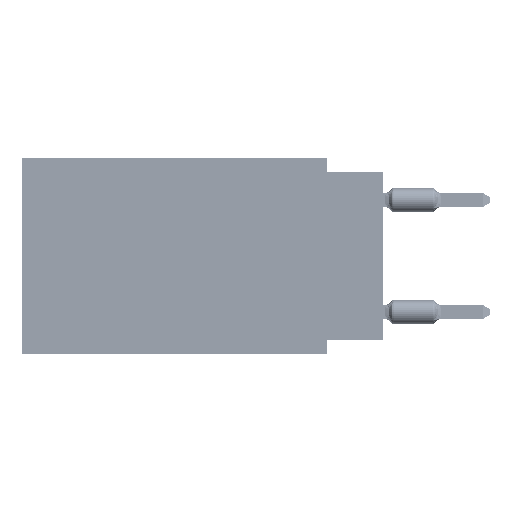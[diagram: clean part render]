
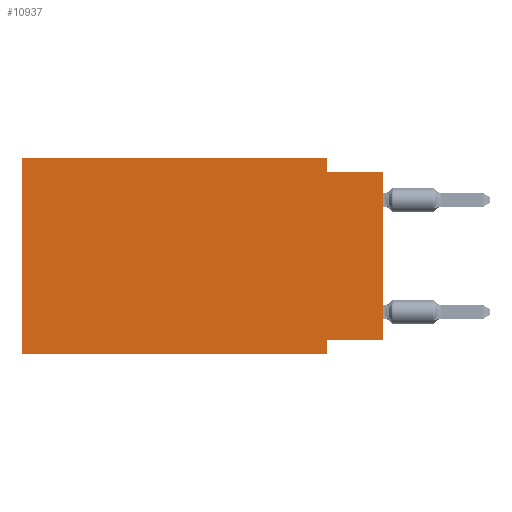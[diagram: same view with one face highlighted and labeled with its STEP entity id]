
A CAD part, left-side view. The second image highlights one B-rep face of the part: STEP entity #10937.
In plain terms, the highlighted planar face has unit normal (-1, 0, 0).
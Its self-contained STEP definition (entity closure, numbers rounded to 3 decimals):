
#2096 = EDGE_CURVE ( 'NONE', #69413, #49470, #41511, .T. ) ;
#5150 = VERTEX_POINT ( 'NONE', #9041 ) ;
#8595 = ORIENTED_EDGE ( 'NONE', *, *, #33761, .F. ) ;
#9041 = CARTESIAN_POINT ( 'NONE',  ( 0., 2.54, 0. ) ) ;
#9292 = CARTESIAN_POINT ( 'NONE',  ( 0., 2.54, -8.89 ) ) ;
#10937 = ADVANCED_FACE ( 'NONE', ( #19559 ), #19094, .F. ) ;
#11481 = DIRECTION ( 'NONE',  ( 0., -1., 0. ) ) ;
#13439 = EDGE_CURVE ( 'NONE', #59198, #5150, #77782, .T. ) ;
#15055 = DIRECTION ( 'NONE',  ( 0., -1., 0. ) ) ;
#19094 = PLANE ( 'NONE',  #81210 ) ;
#19559 = FACE_OUTER_BOUND ( 'NONE', #87181, .T. ) ;
#19826 = ORIENTED_EDGE ( 'NONE', *, *, #53532, .F. ) ;
#23833 = LINE ( 'NONE', #9292, #80689 ) ;
#25296 = EDGE_CURVE ( 'NONE', #86383, #49470, #42517, .T. ) ;
#27376 = CARTESIAN_POINT ( 'NONE',  ( 0., 2.54, -8.255 ) ) ;
#29003 = CARTESIAN_POINT ( 'NONE',  ( 0., 16.383, 0. ) ) ;
#30068 = ORIENTED_EDGE ( 'NONE', *, *, #61194, .F. ) ;
#30643 = CARTESIAN_POINT ( 'NONE',  ( 0., 16.383, 0. ) ) ;
#30698 = ORIENTED_EDGE ( 'NONE', *, *, #2096, .F. ) ;
#33761 = EDGE_CURVE ( 'NONE', #83936, #74518, #23833, .T. ) ;
#34122 = DIRECTION ( 'NONE',  ( 1., 0., 0. ) ) ;
#34676 = VECTOR ( 'NONE', #11481, 1000. ) ;
#35141 = VECTOR ( 'NONE', #36048, 1000. ) ;
#35944 = VECTOR ( 'NONE', #39991, 1000. ) ;
#36048 = DIRECTION ( 'NONE',  ( 0., -1., 0. ) ) ;
#36939 = LINE ( 'NONE', #51019, #76910 ) ;
#37911 = DIRECTION ( 'NONE',  ( 0., 0., -1. ) ) ;
#38393 = ORIENTED_EDGE ( 'NONE', *, *, #88947, .T. ) ;
#39991 = DIRECTION ( 'NONE',  ( 0., 0., 1. ) ) ;
#40229 = DIRECTION ( 'NONE',  ( 0., 0., -1. ) ) ;
#41511 = LINE ( 'NONE', #68247, #34676 ) ;
#42517 = LINE ( 'NONE', #62228, #92619 ) ;
#44725 = ORIENTED_EDGE ( 'NONE', *, *, #52318, .F. ) ;
#48160 = VECTOR ( 'NONE', #15055, 1000. ) ;
#48427 = CARTESIAN_POINT ( 'NONE',  ( 0., 2.54, -0.635 ) ) ;
#49470 = VERTEX_POINT ( 'NONE', #79750 ) ;
#49771 = CARTESIAN_POINT ( 'NONE',  ( 0., 0., -8.255 ) ) ;
#50237 = LINE ( 'NONE', #49771, #53106 ) ;
#51019 = CARTESIAN_POINT ( 'NONE',  ( 0., 2.54, 0. ) ) ;
#52318 = EDGE_CURVE ( 'NONE', #5150, #69413, #36939, .T. ) ;
#53106 = VECTOR ( 'NONE', #78336, 1000. ) ;
#53532 = EDGE_CURVE ( 'NONE', #86383, #83936, #50237, .T. ) ;
#53616 = LINE ( 'NONE', #30643, #35944 ) ;
#57539 = CARTESIAN_POINT ( 'NONE',  ( 0., 16.383, -8.89 ) ) ;
#59198 = VERTEX_POINT ( 'NONE', #62801 ) ;
#61194 = EDGE_CURVE ( 'NONE', #89259, #59198, #53616, .T. ) ;
#62228 = CARTESIAN_POINT ( 'NONE',  ( 0., 0., 0. ) ) ;
#62705 = CARTESIAN_POINT ( 'NONE',  ( 0., 0., -8.255 ) ) ;
#62801 = CARTESIAN_POINT ( 'NONE',  ( 0., 16.383, 0. ) ) ;
#63164 = DIRECTION ( 'NONE',  ( 0., 0., 1. ) ) ;
#65543 = DIRECTION ( 'NONE',  ( 0., 0., -1. ) ) ;
#68247 = CARTESIAN_POINT ( 'NONE',  ( 0., 0., -0.635 ) ) ;
#69280 = CARTESIAN_POINT ( 'NONE',  ( 0., 16.383, 0. ) ) ;
#69413 = VERTEX_POINT ( 'NONE', #48427 ) ;
#74518 = VERTEX_POINT ( 'NONE', #82343 ) ;
#76461 = ORIENTED_EDGE ( 'NONE', *, *, #13439, .F. ) ;
#76910 = VECTOR ( 'NONE', #65543, 1000. ) ;
#77782 = LINE ( 'NONE', #29003, #35141 ) ;
#78336 = DIRECTION ( 'NONE',  ( 0., 1., 0. ) ) ;
#79293 = LINE ( 'NONE', #85858, #48160 ) ;
#79750 = CARTESIAN_POINT ( 'NONE',  ( 0., 0., -0.635 ) ) ;
#80689 = VECTOR ( 'NONE', #37911, 1000. ) ;
#81210 = AXIS2_PLACEMENT_3D ( 'NONE', #69280, #34122, #40229 ) ;
#81408 = ORIENTED_EDGE ( 'NONE', *, *, #25296, .T. ) ;
#82343 = CARTESIAN_POINT ( 'NONE',  ( 0., 2.54, -8.89 ) ) ;
#83936 = VERTEX_POINT ( 'NONE', #27376 ) ;
#85858 = CARTESIAN_POINT ( 'NONE',  ( 0., 16.383, -8.89 ) ) ;
#86383 = VERTEX_POINT ( 'NONE', #62705 ) ;
#87181 = EDGE_LOOP ( 'NONE', ( #81408, #30698, #44725, #76461, #30068, #38393, #8595, #19826 ) ) ;
#88947 = EDGE_CURVE ( 'NONE', #89259, #74518, #79293, .T. ) ;
#89259 = VERTEX_POINT ( 'NONE', #57539 ) ;
#92619 = VECTOR ( 'NONE', #63164, 1000. ) ;
